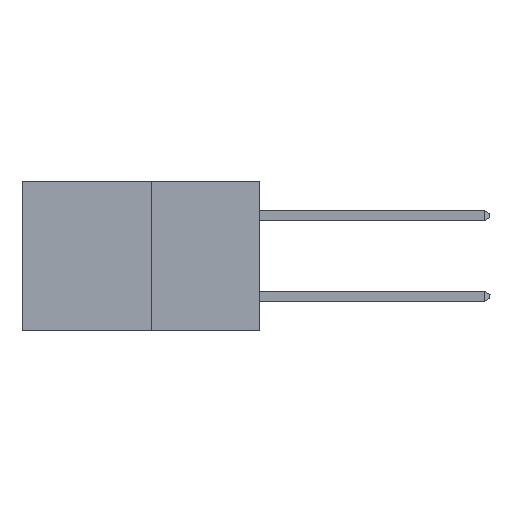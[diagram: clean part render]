
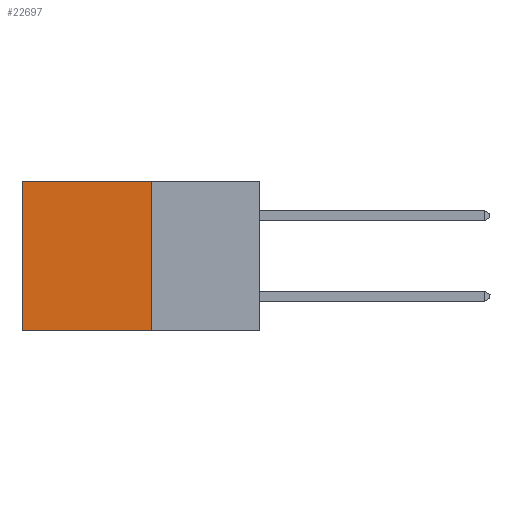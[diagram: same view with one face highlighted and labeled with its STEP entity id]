
A CAD part, left-side view. The second image highlights one B-rep face of the part: STEP entity #22697.
In plain terms, the highlighted planar face has unit normal (-1, 0, 0).
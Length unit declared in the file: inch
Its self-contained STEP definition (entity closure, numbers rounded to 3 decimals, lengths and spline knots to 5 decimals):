
#2433 = AXIS2_PLACEMENT_3D ( 'NONE', #22708, #8515, #21012 ) ;
#2557 = LINE ( 'NONE', #10469, #20642 ) ;
#3690 = DIRECTION ( 'NONE',  ( 0., 0., -1. ) ) ;
#4949 = CARTESIAN_POINT ( 'NONE',  ( 0.277, 0.59, 0. ) ) ;
#5969 = VERTEX_POINT ( 'NONE', #16401 ) ;
#6748 = ORIENTED_EDGE ( 'NONE', *, *, #20812, .F. ) ;
#6787 = DIRECTION ( 'NONE',  ( 0., 1., 0. ) ) ;
#6932 = EDGE_CURVE ( 'NONE', #22000, #21882, #16009, .T. ) ;
#7015 = ORIENTED_EDGE ( 'NONE', *, *, #12303, .T. ) ;
#8515 = DIRECTION ( 'NONE',  ( 1., 0., 0. ) ) ;
#9158 = VECTOR ( 'NONE', #19395, 39.37008 ) ;
#9994 = EDGE_LOOP ( 'NONE', ( #7015, #21804, #6748, #13136 ) ) ;
#10005 = FACE_OUTER_BOUND ( 'NONE', #9994, .T. ) ;
#10469 = CARTESIAN_POINT ( 'NONE',  ( 0.277, 0.27, -0.37 ) ) ;
#12277 = CARTESIAN_POINT ( 'NONE',  ( 0.277, 0.27, 0. ) ) ;
#12303 = EDGE_CURVE ( 'NONE', #21882, #5969, #14001, .T. ) ;
#12903 = CARTESIAN_POINT ( 'NONE',  ( 0.277, 0.27, -0.37 ) ) ;
#13136 = ORIENTED_EDGE ( 'NONE', *, *, #6932, .T. ) ;
#14001 = LINE ( 'NONE', #21137, #9158 ) ;
#14418 = VERTEX_POINT ( 'NONE', #22689 ) ;
#15916 = DIRECTION ( 'NONE',  ( 0., 1., 0. ) ) ;
#16009 = LINE ( 'NONE', #17634, #21195 ) ;
#16401 = CARTESIAN_POINT ( 'NONE',  ( 0.277, 0.59, -0.37 ) ) ;
#17634 = CARTESIAN_POINT ( 'NONE',  ( 0.277, 0.27, 0. ) ) ;
#19020 = LINE ( 'NONE', #12903, #23112 ) ;
#19258 = PLANE ( 'NONE',  #2433 ) ;
#19395 = DIRECTION ( 'NONE',  ( 0., 0., -1. ) ) ;
#20642 = VECTOR ( 'NONE', #15916, 39.37008 ) ;
#20812 = EDGE_CURVE ( 'NONE', #22000, #14418, #19020, .T. ) ;
#21012 = DIRECTION ( 'NONE',  ( 0., 0., -1. ) ) ;
#21137 = CARTESIAN_POINT ( 'NONE',  ( 0.277, 0.59, -0.37 ) ) ;
#21142 = EDGE_CURVE ( 'NONE', #14418, #5969, #2557, .T. ) ;
#21195 = VECTOR ( 'NONE', #6787, 39.37008 ) ;
#21804 = ORIENTED_EDGE ( 'NONE', *, *, #21142, .F. ) ;
#21882 = VERTEX_POINT ( 'NONE', #4949 ) ;
#22000 = VERTEX_POINT ( 'NONE', #12277 ) ;
#22689 = CARTESIAN_POINT ( 'NONE',  ( 0.277, 0.27, -0.37 ) ) ;
#22697 = ADVANCED_FACE ( 'NONE', ( #10005 ), #19258, .F. ) ;
#22708 = CARTESIAN_POINT ( 'NONE',  ( 0.277, 0.27, -0.37 ) ) ;
#23112 = VECTOR ( 'NONE', #3690, 39.37008 ) ;
